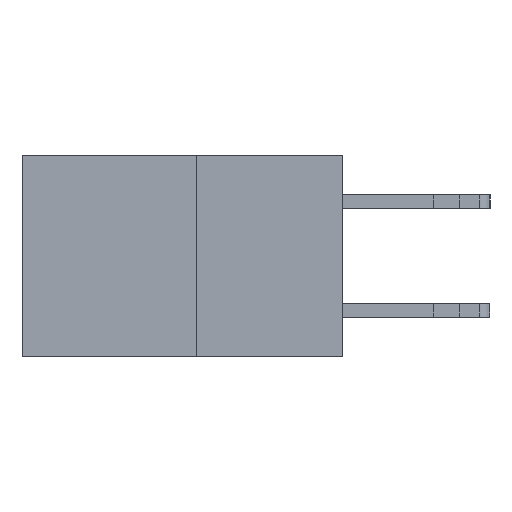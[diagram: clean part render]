
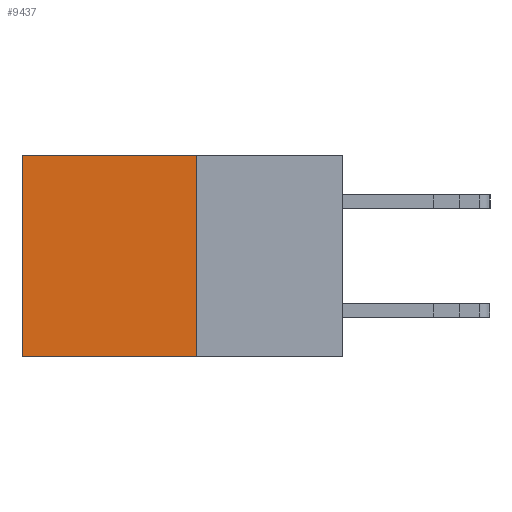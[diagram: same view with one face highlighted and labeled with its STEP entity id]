
A CAD part, left-side view. The second image highlights one B-rep face of the part: STEP entity #9437.
In plain terms, the highlighted planar face has unit normal (-1, 0, 0).
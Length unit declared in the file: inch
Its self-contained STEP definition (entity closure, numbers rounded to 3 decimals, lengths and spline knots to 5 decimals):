
#2793 = DIRECTION ( 'NONE',  ( 0., 0., -1. ) ) ;
#3409 = EDGE_LOOP ( 'NONE', ( #15078, #6133, #17883, #19656 ) ) ;
#5170 = CARTESIAN_POINT ( 'NONE',  ( 0.277, 0.27, -0.37 ) ) ;
#6133 = ORIENTED_EDGE ( 'NONE', *, *, #27333, .F. ) ;
#6447 = AXIS2_PLACEMENT_3D ( 'NONE', #24207, #26542, #12581 ) ;
#7678 = CARTESIAN_POINT ( 'NONE',  ( 0.277, 0.27, 0. ) ) ;
#7908 = PLANE ( 'NONE',  #6447 ) ;
#8067 = LINE ( 'NONE', #5170, #20460 ) ;
#8261 = LINE ( 'NONE', #13426, #26115 ) ;
#9437 = ADVANCED_FACE ( 'NONE', ( #13838 ), #7908, .F. ) ;
#9914 = LINE ( 'NONE', #16719, #16107 ) ;
#9996 = DIRECTION ( 'NONE',  ( 0., 1., 0. ) ) ;
#12581 = DIRECTION ( 'NONE',  ( 0., 0., -1. ) ) ;
#12777 = CARTESIAN_POINT ( 'NONE',  ( 0.277, 0.59, -0.37 ) ) ;
#13426 = CARTESIAN_POINT ( 'NONE',  ( 0.277, 0.27, -0.37 ) ) ;
#13838 = FACE_OUTER_BOUND ( 'NONE', #3409, .T. ) ;
#13996 = VECTOR ( 'NONE', #9996, 39.37008 ) ;
#14613 = CARTESIAN_POINT ( 'NONE',  ( 0.277, 0.27, -0.37 ) ) ;
#15078 = ORIENTED_EDGE ( 'NONE', *, *, #26556, .T. ) ;
#16107 = VECTOR ( 'NONE', #2793, 39.37008 ) ;
#16661 = VERTEX_POINT ( 'NONE', #17706 ) ;
#16719 = CARTESIAN_POINT ( 'NONE',  ( 0.277, 0.59, -0.37 ) ) ;
#17434 = CARTESIAN_POINT ( 'NONE',  ( 0.277, 0.59, 0. ) ) ;
#17706 = CARTESIAN_POINT ( 'NONE',  ( 0.277, 0.27, 0. ) ) ;
#17883 = ORIENTED_EDGE ( 'NONE', *, *, #23505, .F. ) ;
#19656 = ORIENTED_EDGE ( 'NONE', *, *, #24616, .T. ) ;
#19906 = VERTEX_POINT ( 'NONE', #17434 ) ;
#20460 = VECTOR ( 'NONE', #21464, 39.37008 ) ;
#21303 = VERTEX_POINT ( 'NONE', #12777 ) ;
#21464 = DIRECTION ( 'NONE',  ( 0., 1., 0. ) ) ;
#22681 = DIRECTION ( 'NONE',  ( 0., 0., -1. ) ) ;
#23505 = EDGE_CURVE ( 'NONE', #16661, #29517, #8261, .T. ) ;
#24207 = CARTESIAN_POINT ( 'NONE',  ( 0.277, 0.27, -0.37 ) ) ;
#24616 = EDGE_CURVE ( 'NONE', #16661, #19906, #27129, .T. ) ;
#26115 = VECTOR ( 'NONE', #22681, 39.37008 ) ;
#26542 = DIRECTION ( 'NONE',  ( 1., 0., 0. ) ) ;
#26556 = EDGE_CURVE ( 'NONE', #19906, #21303, #9914, .T. ) ;
#27129 = LINE ( 'NONE', #7678, #13996 ) ;
#27333 = EDGE_CURVE ( 'NONE', #29517, #21303, #8067, .T. ) ;
#29517 = VERTEX_POINT ( 'NONE', #14613 ) ;
